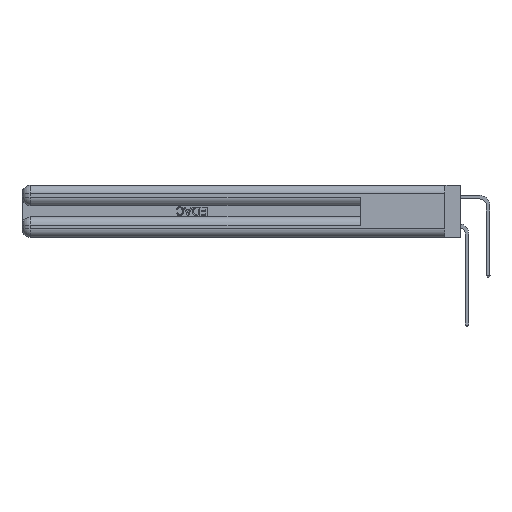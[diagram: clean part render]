
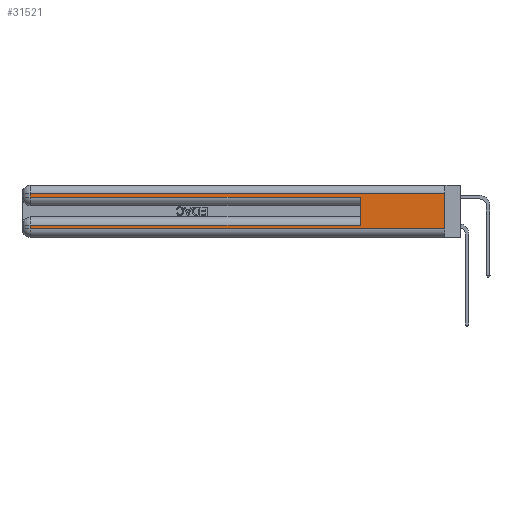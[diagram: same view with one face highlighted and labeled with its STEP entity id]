
A CAD part, left-side view. The second image highlights one B-rep face of the part: STEP entity #31521.
In plain terms, the highlighted planar face has unit normal (-1, 0, 0).
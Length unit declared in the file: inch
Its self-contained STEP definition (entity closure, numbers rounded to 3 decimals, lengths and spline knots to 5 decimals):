
#774 = VERTEX_POINT ( 'NONE', #10559 ) ;
#815 = VERTEX_POINT ( 'NONE', #35095 ) ;
#1972 = EDGE_CURVE ( 'NONE', #28137, #815, #41611, .T. ) ;
#4004 = ORIENTED_EDGE ( 'NONE', *, *, #19741, .T. ) ;
#5236 = VECTOR ( 'NONE', #23763, 39.37008 ) ;
#5589 = LINE ( 'NONE', #33345, #23121 ) ;
#5904 = DIRECTION ( 'NONE',  ( 0., 1., 0. ) ) ;
#6280 = CARTESIAN_POINT ( 'NONE',  ( 0., 0., 0.37 ) ) ;
#6919 = LINE ( 'NONE', #13175, #15225 ) ;
#7833 = VERTEX_POINT ( 'NONE', #8548 ) ;
#8468 = ORIENTED_EDGE ( 'NONE', *, *, #43337, .T. ) ;
#8548 = CARTESIAN_POINT ( 'NONE',  ( 0., 0., 0.31 ) ) ;
#10559 = CARTESIAN_POINT ( 'NONE',  ( 0., 2.94, 0.085 ) ) ;
#10596 = LINE ( 'NONE', #31335, #37149 ) ;
#10642 = DIRECTION ( 'NONE',  ( 0., -1., 0. ) ) ;
#10907 = ORIENTED_EDGE ( 'NONE', *, *, #17394, .F. ) ;
#12396 = VERTEX_POINT ( 'NONE', #26678 ) ;
#13175 = CARTESIAN_POINT ( 'NONE',  ( 0., 0., 0.085 ) ) ;
#13391 = DIRECTION ( 'NONE',  ( 0., 0., -1. ) ) ;
#15225 = VECTOR ( 'NONE', #5904, 39.37008 ) ;
#16386 = LINE ( 'NONE', #17826, #24513 ) ;
#17394 = EDGE_CURVE ( 'NONE', #7833, #35344, #40350, .T. ) ;
#17826 = CARTESIAN_POINT ( 'NONE',  ( 0., 0., 0.31 ) ) ;
#18953 = ORIENTED_EDGE ( 'NONE', *, *, #20745, .T. ) ;
#19683 = VECTOR ( 'NONE', #10642, 39.37008 ) ;
#19741 = EDGE_CURVE ( 'NONE', #12396, #35344, #28895, .T. ) ;
#20453 = CARTESIAN_POINT ( 'NONE',  ( 0., 2.94, 0.37 ) ) ;
#20616 = DIRECTION ( 'NONE',  ( 1., 0., 0. ) ) ;
#20745 = EDGE_CURVE ( 'NONE', #28137, #774, #6919, .T. ) ;
#21313 = DIRECTION ( 'NONE',  ( 0., 1., 0. ) ) ;
#21862 = CARTESIAN_POINT ( 'NONE',  ( 0., 0.6, 0.145 ) ) ;
#22118 = CARTESIAN_POINT ( 'NONE',  ( 0., 2.94, 0.31 ) ) ;
#22173 = ORIENTED_EDGE ( 'NONE', *, *, #1972, .F. ) ;
#22204 = FACE_OUTER_BOUND ( 'NONE', #25510, .T. ) ;
#23121 = VECTOR ( 'NONE', #36808, 39.37008 ) ;
#23763 = DIRECTION ( 'NONE',  ( 0., 0., -1. ) ) ;
#24513 = VECTOR ( 'NONE', #21313, 39.37008 ) ;
#24536 = CARTESIAN_POINT ( 'NONE',  ( 0., 0., 0.06 ) ) ;
#24613 = ORIENTED_EDGE ( 'NONE', *, *, #38641, .T. ) ;
#25196 = DIRECTION ( 'NONE',  ( 0., 0., 1. ) ) ;
#25510 = EDGE_LOOP ( 'NONE', ( #10907, #33324, #24613, #8468, #22173, #18953, #35626, #4004 ) ) ;
#26029 = EDGE_CURVE ( 'NONE', #774, #12396, #34079, .T. ) ;
#26678 = CARTESIAN_POINT ( 'NONE',  ( 0., 2.94, 0.06 ) ) ;
#26714 = VERTEX_POINT ( 'NONE', #22118 ) ;
#28137 = VERTEX_POINT ( 'NONE', #35457 ) ;
#28895 = LINE ( 'NONE', #24536, #19683 ) ;
#31234 = VECTOR ( 'NONE', #13391, 39.37008 ) ;
#31335 = CARTESIAN_POINT ( 'NONE',  ( 0., 0., 0.285 ) ) ;
#31510 = CARTESIAN_POINT ( 'NONE',  ( 0., 2.94, 0.285 ) ) ;
#31521 = ADVANCED_FACE ( 'NONE', ( #22204 ), #37763, .F. ) ;
#33324 = ORIENTED_EDGE ( 'NONE', *, *, #35669, .T. ) ;
#33345 = CARTESIAN_POINT ( 'NONE',  ( 0., 2.94, 0.37 ) ) ;
#33531 = VECTOR ( 'NONE', #25196, 39.37008 ) ;
#34071 = AXIS2_PLACEMENT_3D ( 'NONE', #41204, #20616, #44671 ) ;
#34079 = LINE ( 'NONE', #20453, #5236 ) ;
#35095 = CARTESIAN_POINT ( 'NONE',  ( 0., 0.6, 0.285 ) ) ;
#35344 = VERTEX_POINT ( 'NONE', #39978 ) ;
#35457 = CARTESIAN_POINT ( 'NONE',  ( 0., 0.6, 0.085 ) ) ;
#35626 = ORIENTED_EDGE ( 'NONE', *, *, #26029, .T. ) ;
#35669 = EDGE_CURVE ( 'NONE', #7833, #26714, #16386, .T. ) ;
#36808 = DIRECTION ( 'NONE',  ( 0., 0., -1. ) ) ;
#37149 = VECTOR ( 'NONE', #38095, 39.37008 ) ;
#37763 = PLANE ( 'NONE',  #34071 ) ;
#37800 = VERTEX_POINT ( 'NONE', #31510 ) ;
#38095 = DIRECTION ( 'NONE',  ( 0., -1., 0. ) ) ;
#38641 = EDGE_CURVE ( 'NONE', #26714, #37800, #5589, .T. ) ;
#39978 = CARTESIAN_POINT ( 'NONE',  ( 0., 0., 0.06 ) ) ;
#40350 = LINE ( 'NONE', #6280, #31234 ) ;
#41204 = CARTESIAN_POINT ( 'NONE',  ( 0., 0., 0.37 ) ) ;
#41611 = LINE ( 'NONE', #21862, #33531 ) ;
#43337 = EDGE_CURVE ( 'NONE', #37800, #815, #10596, .T. ) ;
#44671 = DIRECTION ( 'NONE',  ( 0., 0., -1. ) ) ;
